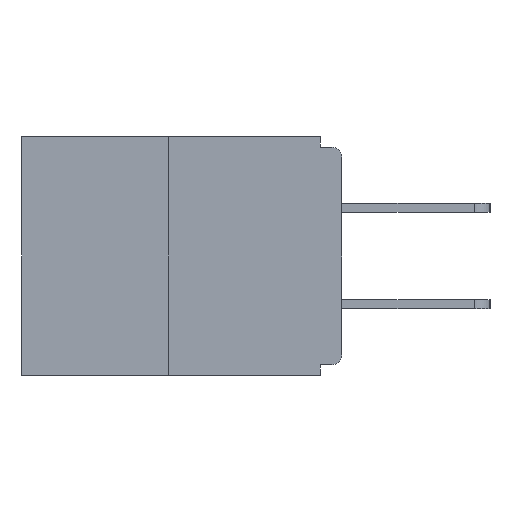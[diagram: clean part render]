
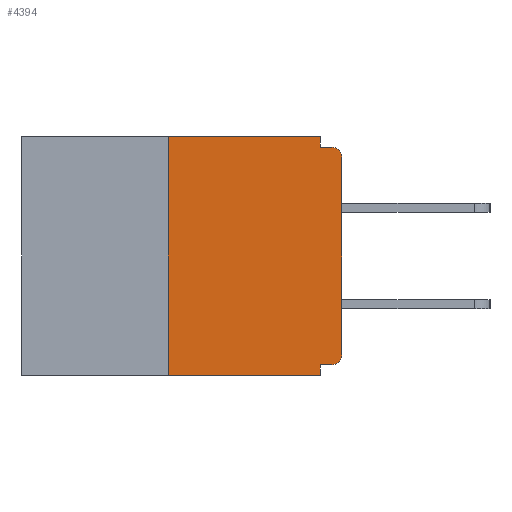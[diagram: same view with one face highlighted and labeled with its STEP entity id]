
A CAD part, left-side view. The second image highlights one B-rep face of the part: STEP entity #4394.
In plain terms, the highlighted planar face has unit normal (-1, 0, 0).
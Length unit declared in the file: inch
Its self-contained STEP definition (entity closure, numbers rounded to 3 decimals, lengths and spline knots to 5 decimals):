
#1289 = EDGE_CURVE ( 'NONE', #11378, #3546, #14825, .T. ) ;
#1401 = DIRECTION ( 'NONE',  ( 0., 0., 1. ) ) ;
#1851 = EDGE_CURVE ( 'NONE', #18853, #9261, #7589, .T. ) ;
#2628 = EDGE_LOOP ( 'NONE', ( #9786, #4413, #18733, #9968, #8938, #23214, #22711, #7920, #21201, #3843 ) ) ;
#2630 = PLANE ( 'NONE',  #24328 ) ;
#2632 = CARTESIAN_POINT ( 'NONE',  ( 0., 0., -0.313 ) ) ;
#2858 = CARTESIAN_POINT ( 'NONE',  ( 0., 0.031, 0. ) ) ;
#3138 = DIRECTION ( 'NONE',  ( 0., 0., 1. ) ) ;
#3546 = VERTEX_POINT ( 'NONE', #15031 ) ;
#3615 = VECTOR ( 'NONE', #1401, 39.37008 ) ;
#3843 = ORIENTED_EDGE ( 'NONE', *, *, #10853, .F. ) ;
#4315 = VECTOR ( 'NONE', #14933, 39.37008 ) ;
#4394 = ADVANCED_FACE ( 'NONE', ( #12401 ), #2630, .F. ) ;
#4413 = ORIENTED_EDGE ( 'NONE', *, *, #1851, .F. ) ;
#4590 = CARTESIAN_POINT ( 'NONE',  ( 0., 0.031, 0. ) ) ;
#4643 = AXIS2_PLACEMENT_3D ( 'NONE', #12718, #14658, #4890 ) ;
#4686 = DIRECTION ( 'NONE',  ( 0., 0., -1. ) ) ;
#4754 = DIRECTION ( 'NONE',  ( 0., 0., -1. ) ) ;
#4890 = DIRECTION ( 'NONE',  ( 0., 0., -1. ) ) ;
#5135 = VERTEX_POINT ( 'NONE', #4590 ) ;
#5307 = CARTESIAN_POINT ( 'NONE',  ( 0., 0.031, -0.015 ) ) ;
#5646 = DIRECTION ( 'NONE',  ( 0., -1., 0. ) ) ;
#5685 = DIRECTION ( 'NONE',  ( -1., 0., 0. ) ) ;
#7353 = CIRCLE ( 'NONE', #4643, 0.015 ) ;
#7404 = DIRECTION ( 'NONE',  ( 0., 0., -1. ) ) ;
#7571 = EDGE_CURVE ( 'NONE', #9261, #5135, #9521, .T. ) ;
#7589 = LINE ( 'NONE', #24915, #3615 ) ;
#7690 = EDGE_CURVE ( 'NONE', #8144, #8625, #7353, .T. ) ;
#7773 = CARTESIAN_POINT ( 'NONE',  ( 0., 0., -0.328 ) ) ;
#7920 = ORIENTED_EDGE ( 'NONE', *, *, #7690, .T. ) ;
#8144 = VERTEX_POINT ( 'NONE', #15208 ) ;
#8625 = VERTEX_POINT ( 'NONE', #17017 ) ;
#8629 = VECTOR ( 'NONE', #5646, 39.37008 ) ;
#8665 = CARTESIAN_POINT ( 'NONE',  ( 0., 0.25, 0. ) ) ;
#8739 = VECTOR ( 'NONE', #14757, 39.37008 ) ;
#8938 = ORIENTED_EDGE ( 'NONE', *, *, #16013, .F. ) ;
#8948 = CARTESIAN_POINT ( 'NONE',  ( 0., 0.031, -0.328 ) ) ;
#9189 = CARTESIAN_POINT ( 'NONE',  ( 0., 0.25, -0.343 ) ) ;
#9261 = VERTEX_POINT ( 'NONE', #8665 ) ;
#9521 = LINE ( 'NONE', #16647, #17790 ) ;
#9786 = ORIENTED_EDGE ( 'NONE', *, *, #7571, .F. ) ;
#9968 = ORIENTED_EDGE ( 'NONE', *, *, #1289, .F. ) ;
#10853 = EDGE_CURVE ( 'NONE', #5135, #14536, #10875, .T. ) ;
#10875 = LINE ( 'NONE', #2858, #12096 ) ;
#11205 = CARTESIAN_POINT ( 'NONE',  ( 0., 0., -0.015 ) ) ;
#11321 = VECTOR ( 'NONE', #3138, 39.37008 ) ;
#11378 = VERTEX_POINT ( 'NONE', #8948 ) ;
#11476 = CARTESIAN_POINT ( 'NONE',  ( 0., 0.015, -0.328 ) ) ;
#12096 = VECTOR ( 'NONE', #4754, 39.37008 ) ;
#12401 = FACE_OUTER_BOUND ( 'NONE', #2628, .T. ) ;
#12718 = CARTESIAN_POINT ( 'NONE',  ( 0., 0.015, -0.03 ) ) ;
#13216 = LINE ( 'NONE', #11205, #4315 ) ;
#14021 = CIRCLE ( 'NONE', #14513, 0.015 ) ;
#14048 = VERTEX_POINT ( 'NONE', #2632 ) ;
#14513 = AXIS2_PLACEMENT_3D ( 'NONE', #21457, #5685, #7404 ) ;
#14536 = VERTEX_POINT ( 'NONE', #5307 ) ;
#14658 = DIRECTION ( 'NONE',  ( -1., 0., 0. ) ) ;
#14757 = DIRECTION ( 'NONE',  ( 0., 0., -1. ) ) ;
#14824 = DIRECTION ( 'NONE',  ( 0., -1., 0. ) ) ;
#14825 = LINE ( 'NONE', #16666, #8739 ) ;
#14933 = DIRECTION ( 'NONE',  ( 0., -1., 0. ) ) ;
#15031 = CARTESIAN_POINT ( 'NONE',  ( 0., 0.031, -0.343 ) ) ;
#15208 = CARTESIAN_POINT ( 'NONE',  ( 0., 0., -0.03 ) ) ;
#15402 = CARTESIAN_POINT ( 'NONE',  ( 0., 0.46, -0.343 ) ) ;
#15413 = EDGE_CURVE ( 'NONE', #18853, #3546, #16573, .T. ) ;
#16013 = EDGE_CURVE ( 'NONE', #25281, #11378, #20595, .T. ) ;
#16439 = CARTESIAN_POINT ( 'NONE',  ( 0., 0.46, 0. ) ) ;
#16512 = LINE ( 'NONE', #16790, #11321 ) ;
#16573 = LINE ( 'NONE', #15402, #8629 ) ;
#16647 = CARTESIAN_POINT ( 'NONE',  ( 0., 0.46, 0. ) ) ;
#16666 = CARTESIAN_POINT ( 'NONE',  ( 0., 0.031, -0.343 ) ) ;
#16790 = CARTESIAN_POINT ( 'NONE',  ( 0., 0., 0. ) ) ;
#17017 = CARTESIAN_POINT ( 'NONE',  ( 0., 0.015, -0.015 ) ) ;
#17790 = VECTOR ( 'NONE', #14824, 39.37008 ) ;
#18733 = ORIENTED_EDGE ( 'NONE', *, *, #15413, .T. ) ;
#18853 = VERTEX_POINT ( 'NONE', #9189 ) ;
#19414 = DIRECTION ( 'NONE',  ( 0., 1., 0. ) ) ;
#20570 = VECTOR ( 'NONE', #19414, 39.37008 ) ;
#20595 = LINE ( 'NONE', #7773, #20570 ) ;
#21201 = ORIENTED_EDGE ( 'NONE', *, *, #24314, .F. ) ;
#21457 = CARTESIAN_POINT ( 'NONE',  ( 0., 0.015, -0.313 ) ) ;
#21654 = EDGE_CURVE ( 'NONE', #14048, #8144, #16512, .T. ) ;
#22421 = DIRECTION ( 'NONE',  ( 1., 0., 0. ) ) ;
#22429 = EDGE_CURVE ( 'NONE', #25281, #14048, #14021, .T. ) ;
#22711 = ORIENTED_EDGE ( 'NONE', *, *, #21654, .T. ) ;
#23214 = ORIENTED_EDGE ( 'NONE', *, *, #22429, .T. ) ;
#24314 = EDGE_CURVE ( 'NONE', #14536, #8625, #13216, .T. ) ;
#24328 = AXIS2_PLACEMENT_3D ( 'NONE', #16439, #22421, #4686 ) ;
#24915 = CARTESIAN_POINT ( 'NONE',  ( 0., 0.25, 0. ) ) ;
#25281 = VERTEX_POINT ( 'NONE', #11476 ) ;
